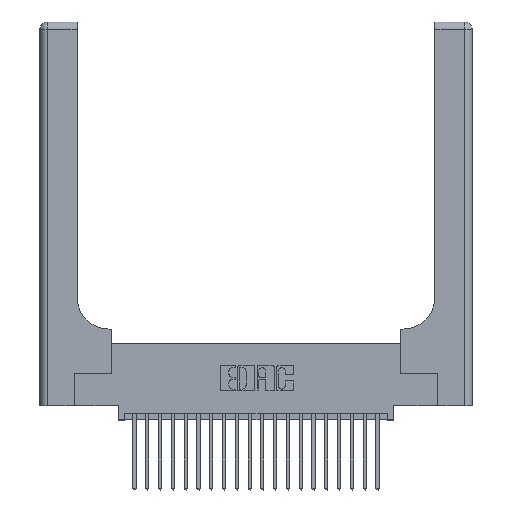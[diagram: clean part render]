
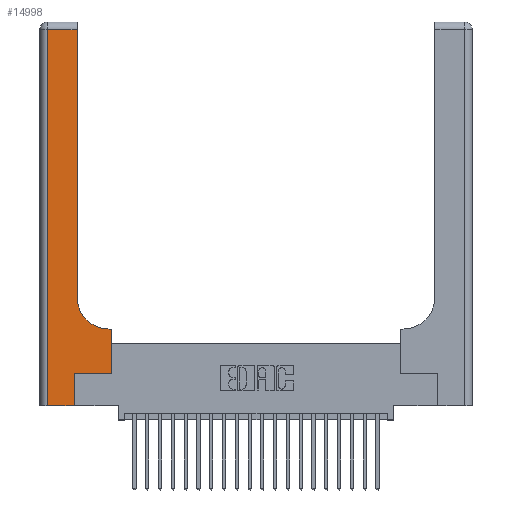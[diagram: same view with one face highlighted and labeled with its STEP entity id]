
A CAD part, top view. The second image highlights one B-rep face of the part: STEP entity #14998.
In plain terms, the highlighted planar face has unit normal (0, 0, 1).
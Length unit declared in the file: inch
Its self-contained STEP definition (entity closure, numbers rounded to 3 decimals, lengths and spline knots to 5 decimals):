
#342 = LINE ( 'NONE', #3653, #4086 ) ;
#637 = VERTEX_POINT ( 'NONE', #18379 ) ;
#1144 = EDGE_CURVE ( 'NONE', #20665, #16940, #5853, .T. ) ;
#2037 = AXIS2_PLACEMENT_3D ( 'NONE', #14057, #10644, #23606 ) ;
#2723 = LINE ( 'NONE', #4354, #10312 ) ;
#3653 = CARTESIAN_POINT ( 'NONE',  ( 0., 2.94, 0.37 ) ) ;
#4086 = VECTOR ( 'NONE', #8953, 39.37008 ) ;
#4275 = LINE ( 'NONE', #12153, #4547 ) ;
#4354 = CARTESIAN_POINT ( 'NONE',  ( 0.2915, 0.6, 0.37 ) ) ;
#4438 = DIRECTION ( 'NONE',  ( 1., 0., 0. ) ) ;
#4461 = ORIENTED_EDGE ( 'NONE', *, *, #8804, .T. ) ;
#4547 = VECTOR ( 'NONE', #13922, 39.37008 ) ;
#4759 = VECTOR ( 'NONE', #11268, 39.37008 ) ;
#4855 = CARTESIAN_POINT ( 'NONE',  ( 0.06, 2.94, 0.37 ) ) ;
#5061 = VECTOR ( 'NONE', #17911, 39.37008 ) ;
#5345 = LINE ( 'NONE', #21642, #5061 ) ;
#5583 = VERTEX_POINT ( 'NONE', #21852 ) ;
#5602 = VERTEX_POINT ( 'NONE', #12629 ) ;
#5709 = EDGE_CURVE ( 'NONE', #637, #23550, #4275, .T. ) ;
#5853 = LINE ( 'NONE', #12872, #15167 ) ;
#6876 = ORIENTED_EDGE ( 'NONE', *, *, #1144, .T. ) ;
#7405 = CARTESIAN_POINT ( 'NONE',  ( 0.06, 0., 0.37 ) ) ;
#8215 = ORIENTED_EDGE ( 'NONE', *, *, #23163, .T. ) ;
#8804 = EDGE_CURVE ( 'NONE', #23211, #637, #12011, .T. ) ;
#8953 = DIRECTION ( 'NONE',  ( -1., 0., 0. ) ) ;
#9287 = ORIENTED_EDGE ( 'NONE', *, *, #15467, .T. ) ;
#9609 = CARTESIAN_POINT ( 'NONE',  ( 0.5585, 0.25, 0.37 ) ) ;
#9909 = ORIENTED_EDGE ( 'NONE', *, *, #20250, .T. ) ;
#10305 = CARTESIAN_POINT ( 'NONE',  ( 0.5415, 0.85, 0.37 ) ) ;
#10312 = VECTOR ( 'NONE', #17177, 39.37008 ) ;
#10569 = FACE_OUTER_BOUND ( 'NONE', #19423, .T. ) ;
#10644 = DIRECTION ( 'NONE',  ( 0., 0., -1. ) ) ;
#10765 = EDGE_CURVE ( 'NONE', #5602, #20665, #342, .T. ) ;
#11026 = CARTESIAN_POINT ( 'NONE',  ( 0.5585, 0.25, 0.37 ) ) ;
#11268 = DIRECTION ( 'NONE',  ( 0., 1., 0. ) ) ;
#11574 = AXIS2_PLACEMENT_3D ( 'NONE', #10305, #23265, #4438 ) ;
#12011 = LINE ( 'NONE', #13230, #16035 ) ;
#12153 = CARTESIAN_POINT ( 'NONE',  ( 0.269, 0.25, 0.37 ) ) ;
#12254 = CARTESIAN_POINT ( 'NONE',  ( 0.269, 0., 0.37 ) ) ;
#12629 = CARTESIAN_POINT ( 'NONE',  ( 0.2915, 2.94, 0.37 ) ) ;
#12872 = CARTESIAN_POINT ( 'NONE',  ( 0.06, 3., 0.37 ) ) ;
#13096 = DIRECTION ( 'NONE',  ( 0., -1., 0. ) ) ;
#13230 = CARTESIAN_POINT ( 'NONE',  ( 0.269, 0., 0.37 ) ) ;
#13231 = LINE ( 'NONE', #16961, #23373 ) ;
#13353 = CARTESIAN_POINT ( 'NONE',  ( 0.5585, 0.6, 0.37 ) ) ;
#13392 = DIRECTION ( 'NONE',  ( 0., 1., 0. ) ) ;
#13922 = DIRECTION ( 'NONE',  ( 1., 0., 0. ) ) ;
#14057 = CARTESIAN_POINT ( 'NONE',  ( 0., 3., 0.37 ) ) ;
#14998 = ADVANCED_FACE ( 'NONE', ( #10569 ), #21657, .F. ) ;
#15167 = VECTOR ( 'NONE', #13096, 39.37008 ) ;
#15467 = EDGE_CURVE ( 'NONE', #21891, #5583, #23074, .T. ) ;
#15523 = LINE ( 'NONE', #9609, #4759 ) ;
#16035 = VECTOR ( 'NONE', #13392, 39.37008 ) ;
#16940 = VERTEX_POINT ( 'NONE', #7405 ) ;
#16961 = CARTESIAN_POINT ( 'NONE',  ( 0., 0., 0.37 ) ) ;
#17177 = DIRECTION ( 'NONE',  ( -1., 0., 0. ) ) ;
#17275 = ORIENTED_EDGE ( 'NONE', *, *, #22804, .T. ) ;
#17911 = DIRECTION ( 'NONE',  ( 0., 1., 0. ) ) ;
#18379 = CARTESIAN_POINT ( 'NONE',  ( 0.269, 0.25, 0.37 ) ) ;
#18903 = ORIENTED_EDGE ( 'NONE', *, *, #10765, .T. ) ;
#19423 = EDGE_LOOP ( 'NONE', ( #20745, #18903, #6876, #17275, #4461, #20851, #9909, #8215, #9287 ) ) ;
#19780 = EDGE_CURVE ( 'NONE', #5583, #5602, #5345, .T. ) ;
#20250 = EDGE_CURVE ( 'NONE', #23550, #20252, #15523, .T. ) ;
#20252 = VERTEX_POINT ( 'NONE', #13353 ) ;
#20665 = VERTEX_POINT ( 'NONE', #4855 ) ;
#20745 = ORIENTED_EDGE ( 'NONE', *, *, #19780, .T. ) ;
#20851 = ORIENTED_EDGE ( 'NONE', *, *, #5709, .T. ) ;
#21642 = CARTESIAN_POINT ( 'NONE',  ( 0.2915, 3., 0.37 ) ) ;
#21657 = PLANE ( 'NONE',  #2037 ) ;
#21852 = CARTESIAN_POINT ( 'NONE',  ( 0.2915, 0.85, 0.37 ) ) ;
#21868 = CARTESIAN_POINT ( 'NONE',  ( 0.5415, 0.6, 0.37 ) ) ;
#21891 = VERTEX_POINT ( 'NONE', #21868 ) ;
#22326 = DIRECTION ( 'NONE',  ( 1., 0., 0. ) ) ;
#22804 = EDGE_CURVE ( 'NONE', #16940, #23211, #13231, .T. ) ;
#23074 = CIRCLE ( 'NONE', #11574, 0.25 ) ;
#23163 = EDGE_CURVE ( 'NONE', #20252, #21891, #2723, .T. ) ;
#23211 = VERTEX_POINT ( 'NONE', #12254 ) ;
#23265 = DIRECTION ( 'NONE',  ( 0., 0., -1. ) ) ;
#23373 = VECTOR ( 'NONE', #22326, 39.37008 ) ;
#23550 = VERTEX_POINT ( 'NONE', #11026 ) ;
#23606 = DIRECTION ( 'NONE',  ( -1., 0., 0. ) ) ;
